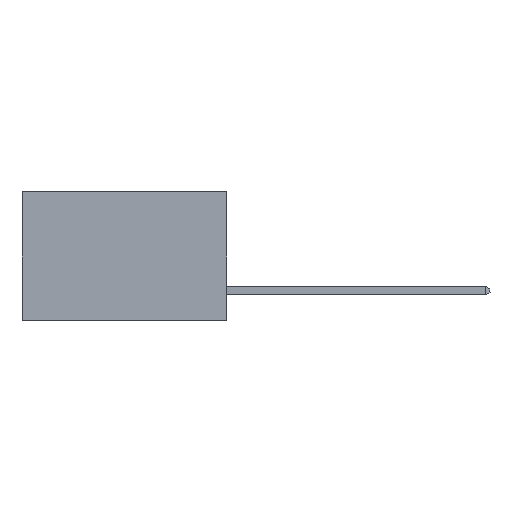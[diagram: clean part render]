
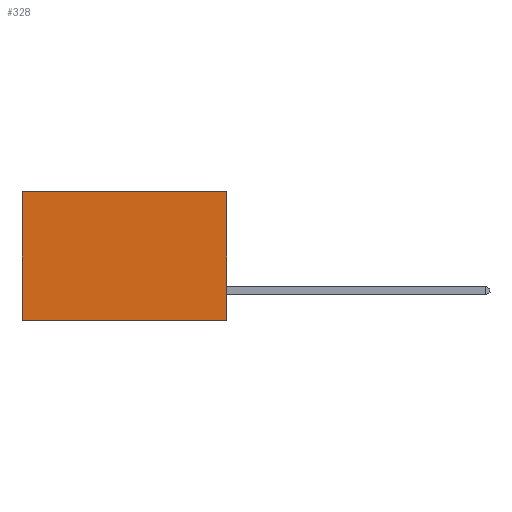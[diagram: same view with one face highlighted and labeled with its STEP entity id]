
A CAD part, left-side view. The second image highlights one B-rep face of the part: STEP entity #328.
In plain terms, the highlighted planar face has unit normal (-1, 0, 0).
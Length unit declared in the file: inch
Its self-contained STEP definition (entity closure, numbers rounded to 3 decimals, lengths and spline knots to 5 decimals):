
#328 = ADVANCED_FACE ( 'NONE', ( #2269 ), #594, .F. ) ;
#594 = PLANE ( 'NONE',  #11340 ) ;
#680 = CARTESIAN_POINT ( 'NONE',  ( 0.277, 0., -0.37 ) ) ;
#915 = CARTESIAN_POINT ( 'NONE',  ( 0.277, 0.59, 0. ) ) ;
#1008 = VERTEX_POINT ( 'NONE', #915 ) ;
#1338 = VERTEX_POINT ( 'NONE', #13437 ) ;
#1466 = CARTESIAN_POINT ( 'NONE',  ( 0.277, 0., 0. ) ) ;
#1478 = DIRECTION ( 'NONE',  ( 1., 0., 0. ) ) ;
#1526 = DIRECTION ( 'NONE',  ( 0., 0., -1. ) ) ;
#1844 = EDGE_CURVE ( 'NONE', #12142, #1008, #11740, .T. ) ;
#1892 = CARTESIAN_POINT ( 'NONE',  ( 0.277, 0., 0. ) ) ;
#1936 = ORIENTED_EDGE ( 'NONE', *, *, #9791, .T. ) ;
#2269 = FACE_OUTER_BOUND ( 'NONE', #3573, .T. ) ;
#2454 = CARTESIAN_POINT ( 'NONE',  ( 0.277, 0., -0.37 ) ) ;
#2687 = VECTOR ( 'NONE', #3141, 39.37008 ) ;
#3141 = DIRECTION ( 'NONE',  ( 0., 1., 0. ) ) ;
#3573 = EDGE_LOOP ( 'NONE', ( #1936, #5152, #8162, #5513 ) ) ;
#3995 = CARTESIAN_POINT ( 'NONE',  ( 0.277, 0., -0.37 ) ) ;
#4104 = VERTEX_POINT ( 'NONE', #14656 ) ;
#5152 = ORIENTED_EDGE ( 'NONE', *, *, #9696, .F. ) ;
#5509 = LINE ( 'NONE', #680, #2687 ) ;
#5513 = ORIENTED_EDGE ( 'NONE', *, *, #1844, .T. ) ;
#6344 = VECTOR ( 'NONE', #7009, 39.37008 ) ;
#7009 = DIRECTION ( 'NONE',  ( 0., 1., 0. ) ) ;
#8162 = ORIENTED_EDGE ( 'NONE', *, *, #9274, .F. ) ;
#8173 = LINE ( 'NONE', #2454, #14283 ) ;
#9086 = DIRECTION ( 'NONE',  ( 0., 0., -1. ) ) ;
#9274 = EDGE_CURVE ( 'NONE', #12142, #1338, #8173, .T. ) ;
#9696 = EDGE_CURVE ( 'NONE', #1338, #4104, #5509, .T. ) ;
#9791 = EDGE_CURVE ( 'NONE', #1008, #4104, #10517, .T. ) ;
#10517 = LINE ( 'NONE', #14780, #13196 ) ;
#11340 = AXIS2_PLACEMENT_3D ( 'NONE', #3995, #1478, #1526 ) ;
#11740 = LINE ( 'NONE', #1892, #6344 ) ;
#12142 = VERTEX_POINT ( 'NONE', #1466 ) ;
#12912 = DIRECTION ( 'NONE',  ( 0., 0., -1. ) ) ;
#13196 = VECTOR ( 'NONE', #9086, 39.37008 ) ;
#13437 = CARTESIAN_POINT ( 'NONE',  ( 0.277, 0., -0.37 ) ) ;
#14283 = VECTOR ( 'NONE', #12912, 39.37008 ) ;
#14656 = CARTESIAN_POINT ( 'NONE',  ( 0.277, 0.59, -0.37 ) ) ;
#14780 = CARTESIAN_POINT ( 'NONE',  ( 0.277, 0.59, -0.37 ) ) ;
